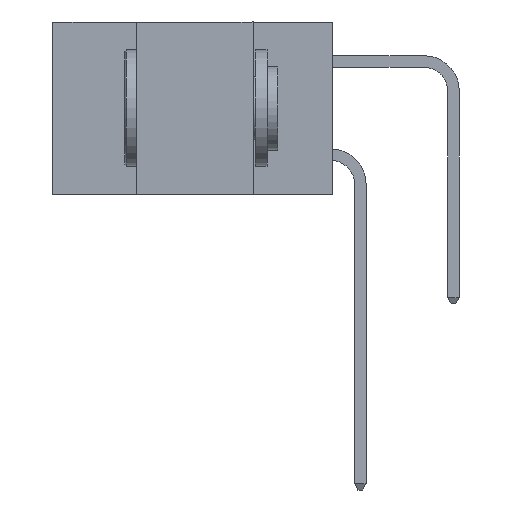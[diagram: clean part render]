
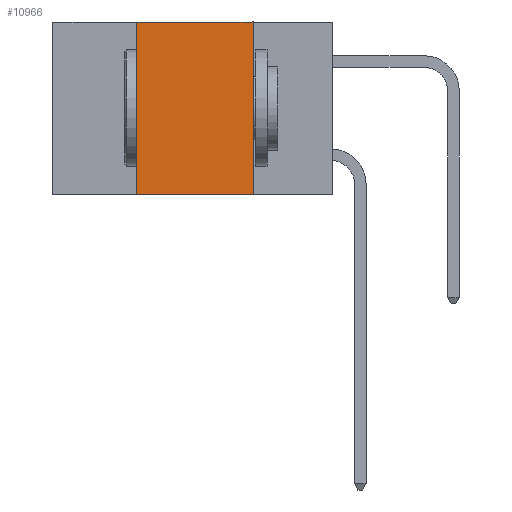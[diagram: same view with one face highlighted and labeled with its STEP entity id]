
A CAD part, left-side view. The second image highlights one B-rep face of the part: STEP entity #10966.
In plain terms, the highlighted planar face has unit normal (-1, 0, 0).
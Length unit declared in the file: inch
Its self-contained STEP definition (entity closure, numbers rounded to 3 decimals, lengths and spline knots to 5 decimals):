
#139 = FACE_OUTER_BOUND ( 'NONE', #10611, .T. ) ;
#206 = EDGE_CURVE ( 'NONE', #1394, #10660, #1035, .T. ) ;
#1035 = LINE ( 'NONE', #4526, #9416 ) ;
#1073 = DIRECTION ( 'NONE',  ( 0., 0., -1. ) ) ;
#1394 = VERTEX_POINT ( 'NONE', #10781 ) ;
#3887 = DIRECTION ( 'NONE',  ( 0., -1., 0. ) ) ;
#3931 = DIRECTION ( 'NONE',  ( 0., -1., 0. ) ) ;
#4526 = CARTESIAN_POINT ( 'NONE',  ( 0., 0.42, -0.37 ) ) ;
#4723 = LINE ( 'NONE', #11608, #13523 ) ;
#5028 = VERTEX_POINT ( 'NONE', #10545 ) ;
#5949 = CARTESIAN_POINT ( 'NONE',  ( 0., 0.42, 0. ) ) ;
#6478 = PLANE ( 'NONE',  #10878 ) ;
#6805 = ORIENTED_EDGE ( 'NONE', *, *, #7299, .F. ) ;
#6874 = VERTEX_POINT ( 'NONE', #9789 ) ;
#6960 = CARTESIAN_POINT ( 'NONE',  ( 0., 0.17, -0.37 ) ) ;
#7053 = DIRECTION ( 'NONE',  ( 0., 0., -1. ) ) ;
#7299 = EDGE_CURVE ( 'NONE', #6874, #5028, #12086, .T. ) ;
#7600 = DIRECTION ( 'NONE',  ( 1., 0., 0. ) ) ;
#7627 = ORIENTED_EDGE ( 'NONE', *, *, #13020, .F. ) ;
#8858 = ORIENTED_EDGE ( 'NONE', *, *, #11257, .T. ) ;
#9416 = VECTOR ( 'NONE', #11779, 39.37008 ) ;
#9501 = VECTOR ( 'NONE', #3887, 39.37008 ) ;
#9595 = CARTESIAN_POINT ( 'NONE',  ( 0., 0.6, 0. ) ) ;
#9789 = CARTESIAN_POINT ( 'NONE',  ( 0., 0.17, 0. ) ) ;
#10545 = CARTESIAN_POINT ( 'NONE',  ( 0., 0.17, -0.37 ) ) ;
#10611 = EDGE_LOOP ( 'NONE', ( #6805, #7627, #11609, #8858 ) ) ;
#10660 = VERTEX_POINT ( 'NONE', #5949 ) ;
#10781 = CARTESIAN_POINT ( 'NONE',  ( 0., 0.42, -0.37 ) ) ;
#10878 = AXIS2_PLACEMENT_3D ( 'NONE', #9595, #7600, #1073 ) ;
#10966 = ADVANCED_FACE ( 'NONE', ( #139 ), #6478, .F. ) ;
#11257 = EDGE_CURVE ( 'NONE', #1394, #5028, #4723, .T. ) ;
#11608 = CARTESIAN_POINT ( 'NONE',  ( 0., 0.6, -0.37 ) ) ;
#11609 = ORIENTED_EDGE ( 'NONE', *, *, #206, .F. ) ;
#11729 = VECTOR ( 'NONE', #7053, 39.37008 ) ;
#11779 = DIRECTION ( 'NONE',  ( 0., 0., 1. ) ) ;
#12086 = LINE ( 'NONE', #6960, #11729 ) ;
#12459 = LINE ( 'NONE', #12712, #9501 ) ;
#12712 = CARTESIAN_POINT ( 'NONE',  ( 0., 0.6, 0. ) ) ;
#13020 = EDGE_CURVE ( 'NONE', #10660, #6874, #12459, .T. ) ;
#13523 = VECTOR ( 'NONE', #3931, 39.37008 ) ;
